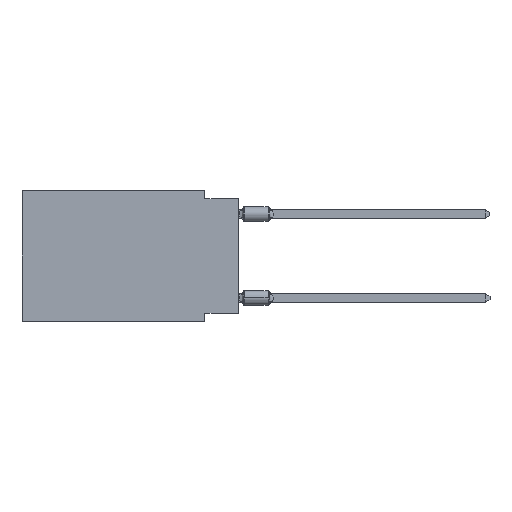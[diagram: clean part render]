
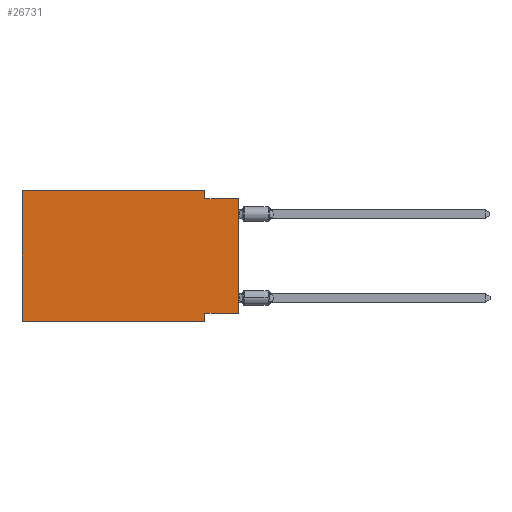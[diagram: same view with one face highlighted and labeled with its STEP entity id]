
A CAD part, left-side view. The second image highlights one B-rep face of the part: STEP entity #26731.
In plain terms, the highlighted planar face has unit normal (-1, 0, 0).
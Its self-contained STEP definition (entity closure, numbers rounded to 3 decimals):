
#122 = EDGE_CURVE ( 'NONE', #10797, #32494, #1960, .T. ) ;
#256 = DIRECTION ( 'NONE',  ( 0., 1., 0. ) ) ;
#529 = ORIENTED_EDGE ( 'NONE', *, *, #17571, .F. ) ;
#580 = VECTOR ( 'NONE', #33018, 1000. ) ;
#1345 = VERTEX_POINT ( 'NONE', #28617 ) ;
#1960 = LINE ( 'NONE', #15535, #25044 ) ;
#3193 = ORIENTED_EDGE ( 'NONE', *, *, #26557, .F. ) ;
#3370 = CARTESIAN_POINT ( 'NONE',  ( 0., 0., -9.271 ) ) ;
#3786 = VECTOR ( 'NONE', #28726, 1000. ) ;
#4428 = AXIS2_PLACEMENT_3D ( 'NONE', #16138, #8392, #24044 ) ;
#4792 = ORIENTED_EDGE ( 'NONE', *, *, #16186, .T. ) ;
#5440 = VECTOR ( 'NONE', #22739, 1000. ) ;
#5569 = LINE ( 'NONE', #6560, #29706 ) ;
#6082 = ORIENTED_EDGE ( 'NONE', *, *, #32997, .F. ) ;
#6451 = DIRECTION ( 'NONE',  ( 0., -1., 0. ) ) ;
#6560 = CARTESIAN_POINT ( 'NONE',  ( 0., 0., -9.271 ) ) ;
#6616 = LINE ( 'NONE', #9207, #32516 ) ;
#8178 = VERTEX_POINT ( 'NONE', #9430 ) ;
#8231 = FACE_OUTER_BOUND ( 'NONE', #27124, .T. ) ;
#8392 = DIRECTION ( 'NONE',  ( 1., 0., 0. ) ) ;
#9207 = CARTESIAN_POINT ( 'NONE',  ( 0., 16.383, 0. ) ) ;
#9430 = CARTESIAN_POINT ( 'NONE',  ( 0., 2.54, -9.271 ) ) ;
#9499 = CARTESIAN_POINT ( 'NONE',  ( 0., 16.383, -9.906 ) ) ;
#10797 = VERTEX_POINT ( 'NONE', #12237 ) ;
#11683 = VERTEX_POINT ( 'NONE', #31692 ) ;
#12237 = CARTESIAN_POINT ( 'NONE',  ( 0., 2.54, 0. ) ) ;
#13217 = ORIENTED_EDGE ( 'NONE', *, *, #28655, .F. ) ;
#13603 = LINE ( 'NONE', #16014, #28797 ) ;
#13769 = DIRECTION ( 'NONE',  ( 0., -1., 0. ) ) ;
#14302 = LINE ( 'NONE', #19446, #18014 ) ;
#14490 = VERTEX_POINT ( 'NONE', #28816 ) ;
#15163 = LINE ( 'NONE', #25649, #3786 ) ;
#15535 = CARTESIAN_POINT ( 'NONE',  ( 0., 2.54, 0. ) ) ;
#16014 = CARTESIAN_POINT ( 'NONE',  ( 0., 0., -0.635 ) ) ;
#16138 = CARTESIAN_POINT ( 'NONE',  ( 0., 16.383, 0. ) ) ;
#16186 = EDGE_CURVE ( 'NONE', #27266, #20386, #14302, .T. ) ;
#17571 = EDGE_CURVE ( 'NONE', #27266, #8178, #5569, .T. ) ;
#18014 = VECTOR ( 'NONE', #26836, 1000. ) ;
#19431 = LINE ( 'NONE', #22541, #580 ) ;
#19446 = CARTESIAN_POINT ( 'NONE',  ( 0., 0., 0. ) ) ;
#19710 = EDGE_CURVE ( 'NONE', #1345, #10797, #6616, .T. ) ;
#20386 = VERTEX_POINT ( 'NONE', #30679 ) ;
#22053 = LINE ( 'NONE', #9499, #5440 ) ;
#22431 = CARTESIAN_POINT ( 'NONE',  ( 0., 2.54, -0.635 ) ) ;
#22541 = CARTESIAN_POINT ( 'NONE',  ( 0., 2.54, -9.906 ) ) ;
#22739 = DIRECTION ( 'NONE',  ( 0., -1., 0. ) ) ;
#23436 = DIRECTION ( 'NONE',  ( 0., 0., -1. ) ) ;
#24044 = DIRECTION ( 'NONE',  ( 0., 0., -1. ) ) ;
#24721 = EDGE_CURVE ( 'NONE', #14490, #11683, #22053, .T. ) ;
#25044 = VECTOR ( 'NONE', #23436, 1000. ) ;
#25220 = ORIENTED_EDGE ( 'NONE', *, *, #24721, .T. ) ;
#25649 = CARTESIAN_POINT ( 'NONE',  ( 0., 16.383, 0. ) ) ;
#26557 = EDGE_CURVE ( 'NONE', #8178, #11683, #19431, .T. ) ;
#26731 = ADVANCED_FACE ( 'NONE', ( #8231 ), #31950, .F. ) ;
#26836 = DIRECTION ( 'NONE',  ( 0., 0., 1. ) ) ;
#27124 = EDGE_LOOP ( 'NONE', ( #4792, #13217, #33799, #32281, #6082, #25220, #3193, #529 ) ) ;
#27266 = VERTEX_POINT ( 'NONE', #3370 ) ;
#28617 = CARTESIAN_POINT ( 'NONE',  ( 0., 16.383, 0. ) ) ;
#28655 = EDGE_CURVE ( 'NONE', #32494, #20386, #13603, .T. ) ;
#28726 = DIRECTION ( 'NONE',  ( 0., 0., 1. ) ) ;
#28797 = VECTOR ( 'NONE', #13769, 1000. ) ;
#28816 = CARTESIAN_POINT ( 'NONE',  ( 0., 16.383, -9.906 ) ) ;
#29706 = VECTOR ( 'NONE', #256, 1000. ) ;
#30679 = CARTESIAN_POINT ( 'NONE',  ( 0., 0., -0.635 ) ) ;
#31692 = CARTESIAN_POINT ( 'NONE',  ( 0., 2.54, -9.906 ) ) ;
#31950 = PLANE ( 'NONE',  #4428 ) ;
#32281 = ORIENTED_EDGE ( 'NONE', *, *, #19710, .F. ) ;
#32494 = VERTEX_POINT ( 'NONE', #22431 ) ;
#32516 = VECTOR ( 'NONE', #6451, 1000. ) ;
#32997 = EDGE_CURVE ( 'NONE', #14490, #1345, #15163, .T. ) ;
#33018 = DIRECTION ( 'NONE',  ( 0., 0., -1. ) ) ;
#33799 = ORIENTED_EDGE ( 'NONE', *, *, #122, .F. ) ;
